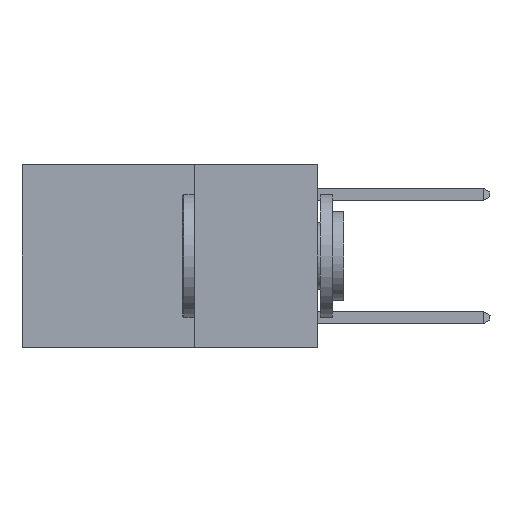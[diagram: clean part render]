
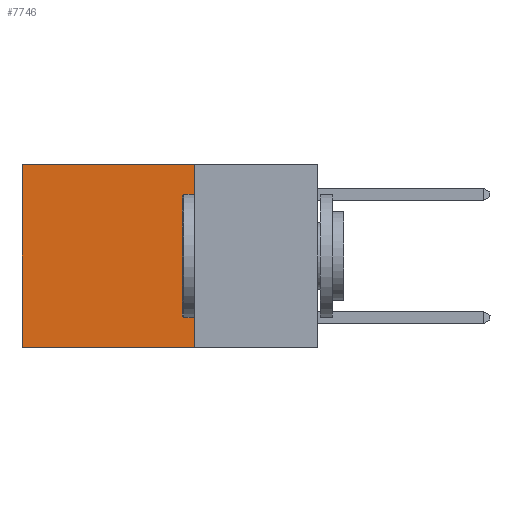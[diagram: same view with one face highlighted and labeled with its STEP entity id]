
A CAD part, left-side view. The second image highlights one B-rep face of the part: STEP entity #7746.
In plain terms, the highlighted planar face has unit normal (-1, 0, 0).
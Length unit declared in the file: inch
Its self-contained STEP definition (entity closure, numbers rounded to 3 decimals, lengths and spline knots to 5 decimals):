
#51 = VERTEX_POINT ( 'NONE', #8964 ) ;
#320 = AXIS2_PLACEMENT_3D ( 'NONE', #16266, #11905, #672 ) ;
#480 = VERTEX_POINT ( 'NONE', #19246 ) ;
#631 = EDGE_CURVE ( 'NONE', #11275, #51, #10362, .T. ) ;
#672 = DIRECTION ( 'NONE',  ( 0., 0., -1. ) ) ;
#845 = CARTESIAN_POINT ( 'NONE',  ( 0.2625, 0.25, 0. ) ) ;
#882 = FACE_OUTER_BOUND ( 'NONE', #4863, .T. ) ;
#1085 = LINE ( 'NONE', #6133, #17333 ) ;
#1726 = CARTESIAN_POINT ( 'NONE',  ( 0.2625, 0.25, 0. ) ) ;
#2076 = LINE ( 'NONE', #845, #17208 ) ;
#4137 = LINE ( 'NONE', #7437, #14729 ) ;
#4863 = EDGE_LOOP ( 'NONE', ( #19060, #7605, #10415, #17861 ) ) ;
#5901 = DIRECTION ( 'NONE',  ( 0., 1., 0. ) ) ;
#6133 = CARTESIAN_POINT ( 'NONE',  ( 0.2625, 0.6, 0. ) ) ;
#7137 = DIRECTION ( 'NONE',  ( 0., 1., 0. ) ) ;
#7437 = CARTESIAN_POINT ( 'NONE',  ( 0.2625, 0.25, -0.37 ) ) ;
#7605 = ORIENTED_EDGE ( 'NONE', *, *, #17393, .F. ) ;
#7746 = ADVANCED_FACE ( 'NONE', ( #882 ), #17699, .F. ) ;
#7895 = EDGE_CURVE ( 'NONE', #480, #8780, #1085, .T. ) ;
#8649 = VECTOR ( 'NONE', #9037, 39.37008 ) ;
#8780 = VERTEX_POINT ( 'NONE', #11487 ) ;
#8964 = CARTESIAN_POINT ( 'NONE',  ( 0.2625, 0.25, -0.37 ) ) ;
#9037 = DIRECTION ( 'NONE',  ( 0., 0., -1. ) ) ;
#10362 = LINE ( 'NONE', #10660, #8649 ) ;
#10415 = ORIENTED_EDGE ( 'NONE', *, *, #631, .F. ) ;
#10660 = CARTESIAN_POINT ( 'NONE',  ( 0.2625, 0.25, 0. ) ) ;
#11275 = VERTEX_POINT ( 'NONE', #1726 ) ;
#11487 = CARTESIAN_POINT ( 'NONE',  ( 0.2625, 0.6, -0.37 ) ) ;
#11905 = DIRECTION ( 'NONE',  ( 1., 0., 0. ) ) ;
#11938 = EDGE_CURVE ( 'NONE', #11275, #480, #2076, .T. ) ;
#14729 = VECTOR ( 'NONE', #5901, 39.37008 ) ;
#16266 = CARTESIAN_POINT ( 'NONE',  ( 0.2625, 0.25, 0. ) ) ;
#17208 = VECTOR ( 'NONE', #7137, 39.37008 ) ;
#17333 = VECTOR ( 'NONE', #19855, 39.37008 ) ;
#17393 = EDGE_CURVE ( 'NONE', #51, #8780, #4137, .T. ) ;
#17699 = PLANE ( 'NONE',  #320 ) ;
#17861 = ORIENTED_EDGE ( 'NONE', *, *, #11938, .T. ) ;
#19060 = ORIENTED_EDGE ( 'NONE', *, *, #7895, .T. ) ;
#19246 = CARTESIAN_POINT ( 'NONE',  ( 0.2625, 0.6, 0. ) ) ;
#19855 = DIRECTION ( 'NONE',  ( 0., 0., -1. ) ) ;
